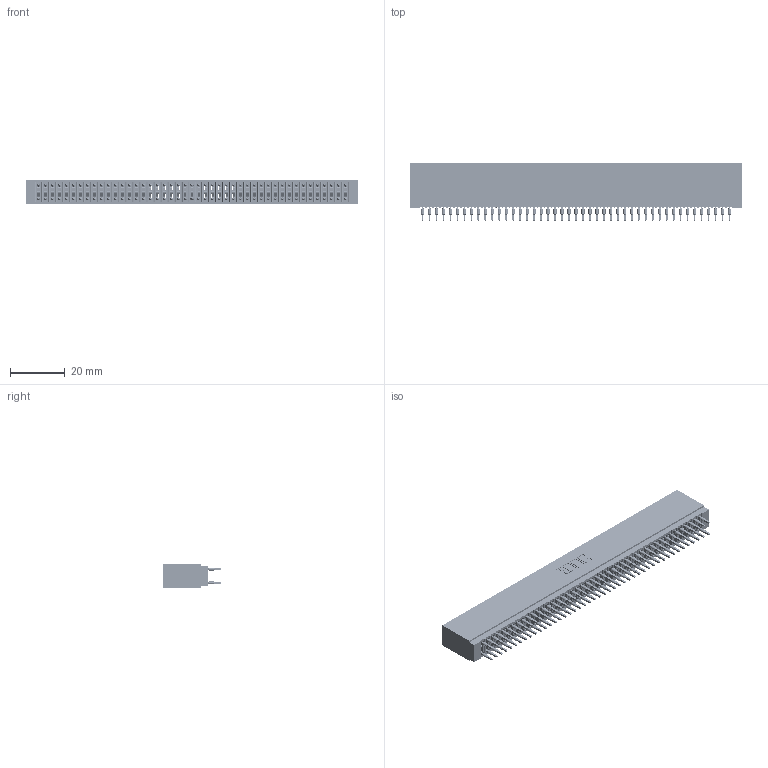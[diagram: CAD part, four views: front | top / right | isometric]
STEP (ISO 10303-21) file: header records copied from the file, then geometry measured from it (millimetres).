
FILE_DESCRIPTION (( 'STEP AP203' ), '1' );
FILE_NAME ('745-090-560-201.STEP', '2020-09-14T11:25:29', ( '' ), ( '' ), 'SwSTEP 2.0', 'SolidWorks 2020', '' );
FILE_SCHEMA (( 'CONFIG_CONTROL_DESIGN' ));
Length unit declared in the file: inch
Products named in the file (3): 745-292-001_560; 745 Part_Insulator Option - 01; 745-090-560-201
Assembly tree (91 placements, depth 2):
  745-090-560-201
    745 Part_Insulator Option - 01
    745-292-001_560  x90
Bounding box: 120.9 x 21.22 x 8.89 mm (x, y, z)
Volume: 11203.5 mm3; surface area: 24264.4 mm2
Topology: 91 solids, 91 shells, 8960 faces, 24513 edges, 15562 vertices
Faces by surface type: plane 4645, cylinder 1975, bspline 1800, torus 540
Entity records: 75678 total; most frequent: CARTESIAN_POINT 13629, ORIENTED_EDGE 13070, DIRECTION 11419, EDGE_CURVE 6535, VECTOR 6075, LINE 6075, VERTEX_POINT 4170, AXIS2_PLACEMENT_3D 2672
